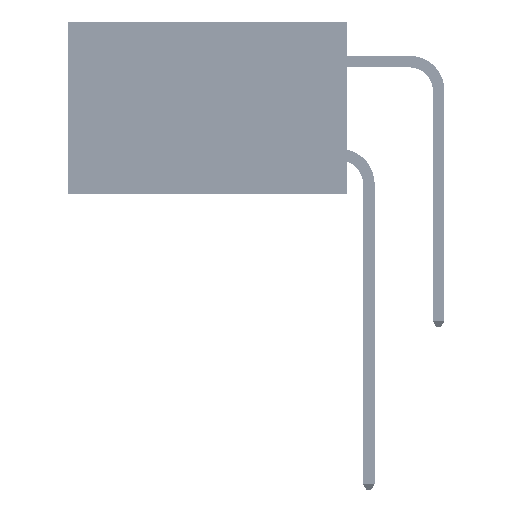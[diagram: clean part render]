
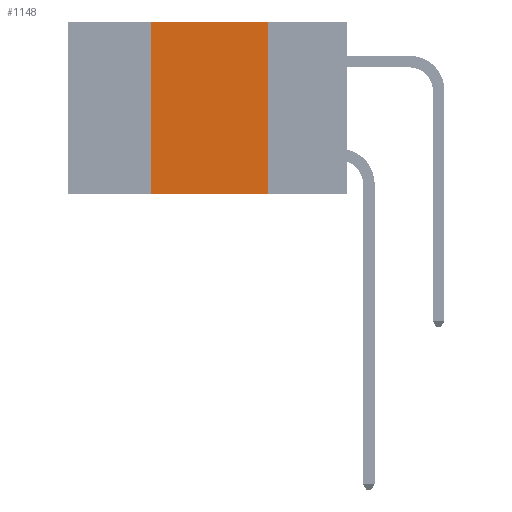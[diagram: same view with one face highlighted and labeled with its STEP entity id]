
A CAD part, left-side view. The second image highlights one B-rep face of the part: STEP entity #1148.
In plain terms, the highlighted planar face has unit normal (-1, 0, 0).
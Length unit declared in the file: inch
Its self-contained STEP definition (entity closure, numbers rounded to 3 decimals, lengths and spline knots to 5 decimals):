
#982 = DIRECTION ( 'NONE',  ( 1., 0., 0. ) ) ;
#1148 = ADVANCED_FACE ( 'NONE', ( #33642 ), #43518, .F. ) ;
#1167 = DIRECTION ( 'NONE',  ( 0., 0., -1. ) ) ;
#2176 = ORIENTED_EDGE ( 'NONE', *, *, #27979, .T. ) ;
#2958 = AXIS2_PLACEMENT_3D ( 'NONE', #51059, #982, #1167 ) ;
#4431 = VECTOR ( 'NONE', #10378, 39.37008 ) ;
#6982 = DIRECTION ( 'NONE',  ( 0., 0., -1. ) ) ;
#9735 = EDGE_CURVE ( 'NONE', #13172, #48571, #30843, .T. ) ;
#10378 = DIRECTION ( 'NONE',  ( 0., -1., 0. ) ) ;
#10833 = CARTESIAN_POINT ( 'NONE',  ( 0., 0.42, 0. ) ) ;
#13172 = VERTEX_POINT ( 'NONE', #37734 ) ;
#15501 = ORIENTED_EDGE ( 'NONE', *, *, #51843, .F. ) ;
#15796 = DIRECTION ( 'NONE',  ( 0., -1., 0. ) ) ;
#17540 = LINE ( 'NONE', #52078, #4431 ) ;
#22585 = LINE ( 'NONE', #36627, #27832 ) ;
#26383 = LINE ( 'NONE', #46254, #36148 ) ;
#27832 = VECTOR ( 'NONE', #15796, 39.37008 ) ;
#27979 = EDGE_CURVE ( 'NONE', #43461, #48571, #17540, .T. ) ;
#28112 = ORIENTED_EDGE ( 'NONE', *, *, #9735, .F. ) ;
#30843 = LINE ( 'NONE', #49639, #38055 ) ;
#30853 = EDGE_CURVE ( 'NONE', #43461, #44298, #26383, .T. ) ;
#33642 = FACE_OUTER_BOUND ( 'NONE', #46285, .T. ) ;
#36148 = VECTOR ( 'NONE', #37667, 39.37008 ) ;
#36627 = CARTESIAN_POINT ( 'NONE',  ( 0., 0.6, 0. ) ) ;
#37667 = DIRECTION ( 'NONE',  ( 0., 0., 1. ) ) ;
#37734 = CARTESIAN_POINT ( 'NONE',  ( 0., 0.17, 0. ) ) ;
#38055 = VECTOR ( 'NONE', #6982, 39.37008 ) ;
#39431 = CARTESIAN_POINT ( 'NONE',  ( 0., 0.17, -0.37 ) ) ;
#42247 = ORIENTED_EDGE ( 'NONE', *, *, #30853, .F. ) ;
#43461 = VERTEX_POINT ( 'NONE', #47134 ) ;
#43518 = PLANE ( 'NONE',  #2958 ) ;
#44298 = VERTEX_POINT ( 'NONE', #10833 ) ;
#46254 = CARTESIAN_POINT ( 'NONE',  ( 0., 0.42, 0. ) ) ;
#46285 = EDGE_LOOP ( 'NONE', ( #28112, #15501, #42247, #2176 ) ) ;
#47134 = CARTESIAN_POINT ( 'NONE',  ( 0., 0.42, -0.37 ) ) ;
#48571 = VERTEX_POINT ( 'NONE', #39431 ) ;
#49639 = CARTESIAN_POINT ( 'NONE',  ( 0., 0.17, 0. ) ) ;
#51059 = CARTESIAN_POINT ( 'NONE',  ( 0., 0.6, 0. ) ) ;
#51843 = EDGE_CURVE ( 'NONE', #44298, #13172, #22585, .T. ) ;
#52078 = CARTESIAN_POINT ( 'NONE',  ( 0., 0.6, -0.37 ) ) ;
